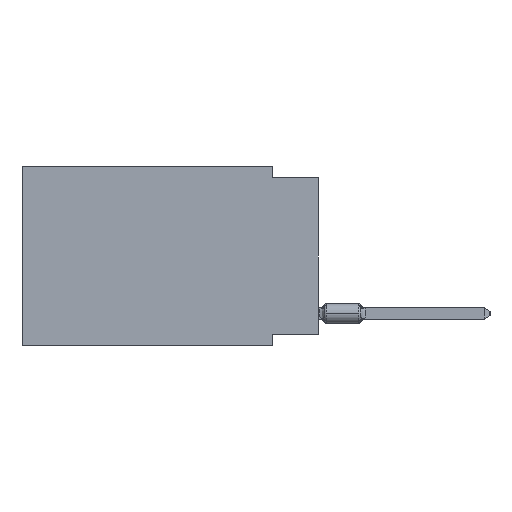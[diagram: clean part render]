
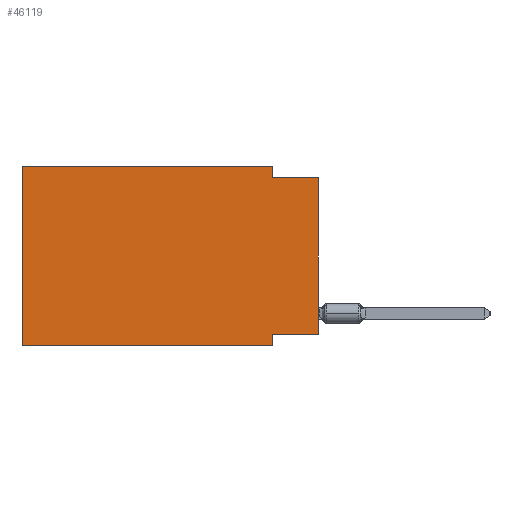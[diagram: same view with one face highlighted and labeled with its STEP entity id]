
A CAD part, left-side view. The second image highlights one B-rep face of the part: STEP entity #46119.
In plain terms, the highlighted planar face has unit normal (-1, 0, 0).
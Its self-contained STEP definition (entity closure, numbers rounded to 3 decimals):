
#390 = CARTESIAN_POINT ( 'NONE',  ( 0., 2.54, 0. ) ) ;
#808 = VERTEX_POINT ( 'NONE', #45908 ) ;
#1035 = EDGE_CURVE ( 'NONE', #3054, #46997, #4245, .T. ) ;
#1299 = DIRECTION ( 'NONE',  ( 0., 0., -1. ) ) ;
#2824 = VERTEX_POINT ( 'NONE', #390 ) ;
#3054 = VERTEX_POINT ( 'NONE', #33472 ) ;
#4245 = LINE ( 'NONE', #27778, #43710 ) ;
#5781 = VECTOR ( 'NONE', #11144, 1000. ) ;
#7285 = VECTOR ( 'NONE', #12879, 1000. ) ;
#8950 = CARTESIAN_POINT ( 'NONE',  ( 0., 16.383, 0. ) ) ;
#9307 = VECTOR ( 'NONE', #36617, 1000. ) ;
#9790 = VECTOR ( 'NONE', #30780, 1000. ) ;
#11144 = DIRECTION ( 'NONE',  ( 0., 1., 0. ) ) ;
#12879 = DIRECTION ( 'NONE',  ( 0., -1., 0. ) ) ;
#13230 = VERTEX_POINT ( 'NONE', #27829 ) ;
#13346 = ORIENTED_EDGE ( 'NONE', *, *, #38447, .F. ) ;
#15342 = EDGE_CURVE ( 'NONE', #16983, #808, #20396, .T. ) ;
#15343 = VECTOR ( 'NONE', #47740, 1000. ) ;
#16983 = VERTEX_POINT ( 'NONE', #19711 ) ;
#17837 = CARTESIAN_POINT ( 'NONE',  ( 0., 2.54, -9.906 ) ) ;
#19170 = LINE ( 'NONE', #31320, #5781 ) ;
#19711 = CARTESIAN_POINT ( 'NONE',  ( 0., 2.54, -0.635 ) ) ;
#20179 = ORIENTED_EDGE ( 'NONE', *, *, #15342, .F. ) ;
#20396 = LINE ( 'NONE', #36158, #7285 ) ;
#21866 = FACE_OUTER_BOUND ( 'NONE', #36990, .T. ) ;
#22120 = DIRECTION ( 'NONE',  ( 0., 0., -1. ) ) ;
#25411 = VERTEX_POINT ( 'NONE', #45322 ) ;
#25810 = VECTOR ( 'NONE', #41514, 1000. ) ;
#26757 = PLANE ( 'NONE',  #47309 ) ;
#27778 = CARTESIAN_POINT ( 'NONE',  ( 0., 16.383, -9.906 ) ) ;
#27829 = CARTESIAN_POINT ( 'NONE',  ( 0., 0., -9.271 ) ) ;
#28498 = ORIENTED_EDGE ( 'NONE', *, *, #42189, .T. ) ;
#28832 = ORIENTED_EDGE ( 'NONE', *, *, #33431, .F. ) ;
#29480 = LINE ( 'NONE', #17837, #39592 ) ;
#30172 = CARTESIAN_POINT ( 'NONE',  ( 0., 2.54, -9.906 ) ) ;
#30774 = LINE ( 'NONE', #32228, #15343 ) ;
#30780 = DIRECTION ( 'NONE',  ( 0., 0., 1. ) ) ;
#31320 = CARTESIAN_POINT ( 'NONE',  ( 0., 0., -9.271 ) ) ;
#31414 = DIRECTION ( 'NONE',  ( 0., -1., 0. ) ) ;
#32228 = CARTESIAN_POINT ( 'NONE',  ( 0., 16.383, 0. ) ) ;
#32985 = ORIENTED_EDGE ( 'NONE', *, *, #37281, .F. ) ;
#33431 = EDGE_CURVE ( 'NONE', #3054, #25411, #30774, .T. ) ;
#33472 = CARTESIAN_POINT ( 'NONE',  ( 0., 16.383, -9.906 ) ) ;
#36158 = CARTESIAN_POINT ( 'NONE',  ( 0., 0., -0.635 ) ) ;
#36617 = DIRECTION ( 'NONE',  ( 0., 0., -1. ) ) ;
#36990 = EDGE_LOOP ( 'NONE', ( #28498, #20179, #50561, #13346, #28832, #43399, #46284, #32985 ) ) ;
#37281 = EDGE_CURVE ( 'NONE', #13230, #46245, #19170, .T. ) ;
#38321 = EDGE_CURVE ( 'NONE', #2824, #16983, #48502, .T. ) ;
#38447 = EDGE_CURVE ( 'NONE', #25411, #2824, #40766, .T. ) ;
#39418 = CARTESIAN_POINT ( 'NONE',  ( 0., 2.54, -9.271 ) ) ;
#39552 = LINE ( 'NONE', #46537, #9790 ) ;
#39592 = VECTOR ( 'NONE', #1299, 1000. ) ;
#40766 = LINE ( 'NONE', #8950, #25810 ) ;
#41514 = DIRECTION ( 'NONE',  ( 0., -1., 0. ) ) ;
#42189 = EDGE_CURVE ( 'NONE', #13230, #808, #39552, .T. ) ;
#43399 = ORIENTED_EDGE ( 'NONE', *, *, #1035, .T. ) ;
#43710 = VECTOR ( 'NONE', #31414, 1000. ) ;
#45322 = CARTESIAN_POINT ( 'NONE',  ( 0., 16.383, 0. ) ) ;
#45382 = CARTESIAN_POINT ( 'NONE',  ( 0., 2.54, 0. ) ) ;
#45648 = CARTESIAN_POINT ( 'NONE',  ( 0., 16.383, 0. ) ) ;
#45908 = CARTESIAN_POINT ( 'NONE',  ( 0., 0., -0.635 ) ) ;
#46119 = ADVANCED_FACE ( 'NONE', ( #21866 ), #26757, .F. ) ;
#46245 = VERTEX_POINT ( 'NONE', #39418 ) ;
#46284 = ORIENTED_EDGE ( 'NONE', *, *, #48971, .F. ) ;
#46537 = CARTESIAN_POINT ( 'NONE',  ( 0., 0., 0. ) ) ;
#46997 = VERTEX_POINT ( 'NONE', #30172 ) ;
#47309 = AXIS2_PLACEMENT_3D ( 'NONE', #45648, #49773, #22120 ) ;
#47740 = DIRECTION ( 'NONE',  ( 0., 0., 1. ) ) ;
#48502 = LINE ( 'NONE', #45382, #9307 ) ;
#48971 = EDGE_CURVE ( 'NONE', #46245, #46997, #29480, .T. ) ;
#49773 = DIRECTION ( 'NONE',  ( 1., 0., 0. ) ) ;
#50561 = ORIENTED_EDGE ( 'NONE', *, *, #38321, .F. ) ;
